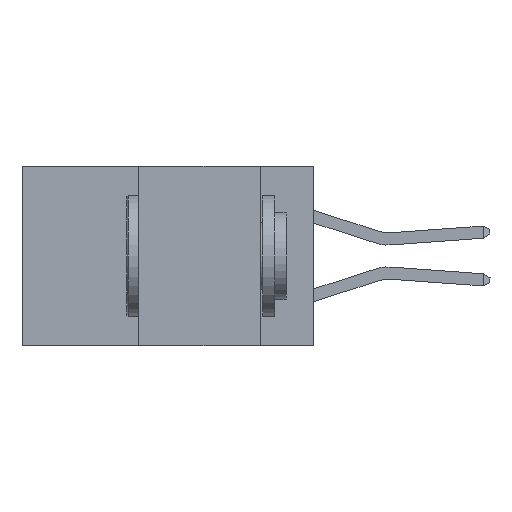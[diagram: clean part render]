
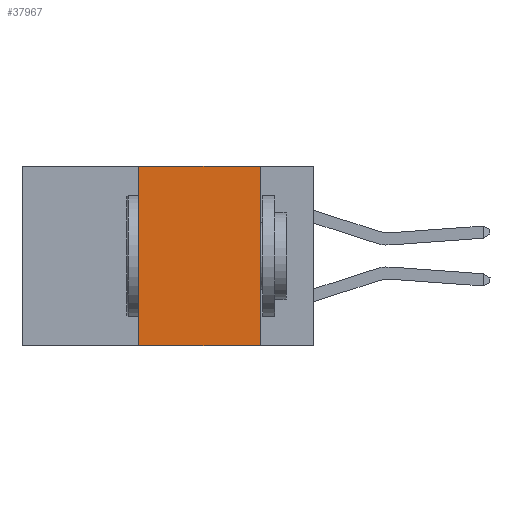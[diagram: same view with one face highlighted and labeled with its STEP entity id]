
A CAD part, left-side view. The second image highlights one B-rep face of the part: STEP entity #37967.
In plain terms, the highlighted planar face has unit normal (-1, 0, 0).
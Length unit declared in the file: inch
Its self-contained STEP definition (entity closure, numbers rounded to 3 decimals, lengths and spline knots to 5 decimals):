
#738 = VERTEX_POINT ( 'NONE', #6096 ) ;
#2175 = LINE ( 'NONE', #41806, #21660 ) ;
#2285 = CARTESIAN_POINT ( 'NONE',  ( 0., 0.6, -0.37 ) ) ;
#2949 = VERTEX_POINT ( 'NONE', #28232 ) ;
#3218 = LINE ( 'NONE', #30812, #33248 ) ;
#3590 = DIRECTION ( 'NONE',  ( 0., 0., -1. ) ) ;
#6096 = CARTESIAN_POINT ( 'NONE',  ( 0., 0.11, -0.37 ) ) ;
#6114 = DIRECTION ( 'NONE',  ( 0., -1., 0. ) ) ;
#7841 = EDGE_CURVE ( 'NONE', #8215, #2949, #2175, .T. ) ;
#8000 = LINE ( 'NONE', #2285, #43323 ) ;
#8215 = VERTEX_POINT ( 'NONE', #19216 ) ;
#9209 = VECTOR ( 'NONE', #30051, 39.37008 ) ;
#10012 = PLANE ( 'NONE',  #33072 ) ;
#15704 = ORIENTED_EDGE ( 'NONE', *, *, #35962, .T. ) ;
#17075 = CARTESIAN_POINT ( 'NONE',  ( 0., 0.6, 0. ) ) ;
#19179 = LINE ( 'NONE', #40381, #9209 ) ;
#19216 = CARTESIAN_POINT ( 'NONE',  ( 0., 0.36, 0. ) ) ;
#19690 = EDGE_CURVE ( 'NONE', #41816, #8215, #19179, .T. ) ;
#21570 = DIRECTION ( 'NONE',  ( 0., -1., 0. ) ) ;
#21660 = VECTOR ( 'NONE', #21570, 39.37008 ) ;
#23131 = ORIENTED_EDGE ( 'NONE', *, *, #7841, .F. ) ;
#24680 = FACE_OUTER_BOUND ( 'NONE', #30721, .T. ) ;
#25509 = EDGE_CURVE ( 'NONE', #2949, #738, #3218, .T. ) ;
#27031 = ORIENTED_EDGE ( 'NONE', *, *, #19690, .F. ) ;
#28232 = CARTESIAN_POINT ( 'NONE',  ( 0., 0.11, 0. ) ) ;
#30051 = DIRECTION ( 'NONE',  ( 0., 0., 1. ) ) ;
#30321 = DIRECTION ( 'NONE',  ( 1., 0., 0. ) ) ;
#30721 = EDGE_LOOP ( 'NONE', ( #42321, #23131, #27031, #15704 ) ) ;
#30812 = CARTESIAN_POINT ( 'NONE',  ( 0., 0.11, 0. ) ) ;
#33072 = AXIS2_PLACEMENT_3D ( 'NONE', #17075, #30321, #33540 ) ;
#33248 = VECTOR ( 'NONE', #3590, 39.37008 ) ;
#33540 = DIRECTION ( 'NONE',  ( 0., 0., -1. ) ) ;
#35962 = EDGE_CURVE ( 'NONE', #41816, #738, #8000, .T. ) ;
#37967 = ADVANCED_FACE ( 'NONE', ( #24680 ), #10012, .F. ) ;
#39218 = CARTESIAN_POINT ( 'NONE',  ( 0., 0.36, -0.37 ) ) ;
#40381 = CARTESIAN_POINT ( 'NONE',  ( 0., 0.36, 0. ) ) ;
#41806 = CARTESIAN_POINT ( 'NONE',  ( 0., 0.6, 0. ) ) ;
#41816 = VERTEX_POINT ( 'NONE', #39218 ) ;
#42321 = ORIENTED_EDGE ( 'NONE', *, *, #25509, .F. ) ;
#43323 = VECTOR ( 'NONE', #6114, 39.37008 ) ;
